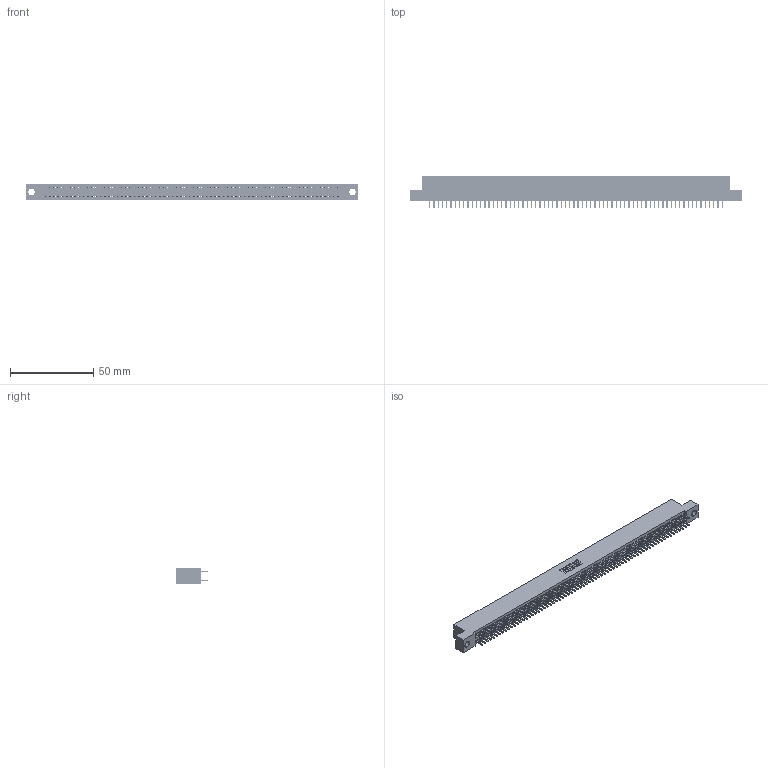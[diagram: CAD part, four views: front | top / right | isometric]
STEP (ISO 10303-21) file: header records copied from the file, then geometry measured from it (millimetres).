
FILE_DESCRIPTION (( 'STEP AP203' ), '1' );
FILE_NAME ('395-140-520-204.STEP', '2018-12-05T19:06:24', ( '' ), ( '' ), 'SwSTEP 2.0', 'SolidWorks 2016', '' );
FILE_SCHEMA (( 'CONFIG_CONTROL_DESIGN' ));
Length unit declared in the file: inch
Products named in the file (3): 345 Part_Flush Mounting Lugs - 0.156 Dia-TH; 395-140-520-204; 345-292-001_345-293-120
Assembly tree (141 placements, depth 2):
  395-140-520-204
    345 Part_Flush Mounting Lugs - 0.156 Dia-TH
    345-292-001_345-293-120  x140
Bounding box: 199.01 x 19.68 x 9.4 mm (x, y, z)
Volume: 19442.4 mm3; surface area: 28965.8 mm2
Topology: 141 solids, 141 shells, 7686 faces, 22321 edges, 14506 vertices
Faces by surface type: plane 4980, cylinder 2706
Entity records: 51271 total; most frequent: CARTESIAN_POINT 8580, ORIENTED_EDGE 8502, DIRECTION 7519, EDGE_CURVE 4251, VECTOR 3835, LINE 3835, VERTEX_POINT 2830, AXIS2_PLACEMENT_3D 1842
